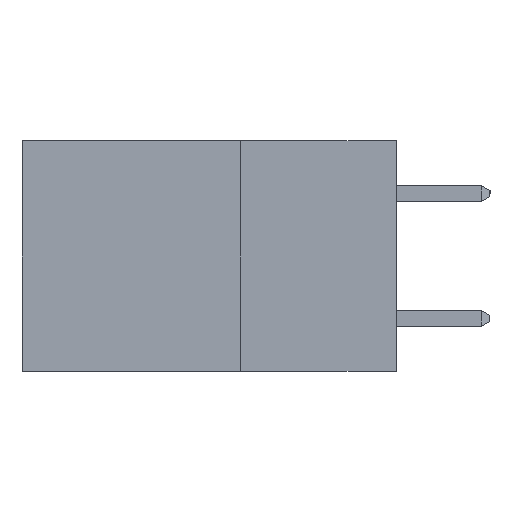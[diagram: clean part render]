
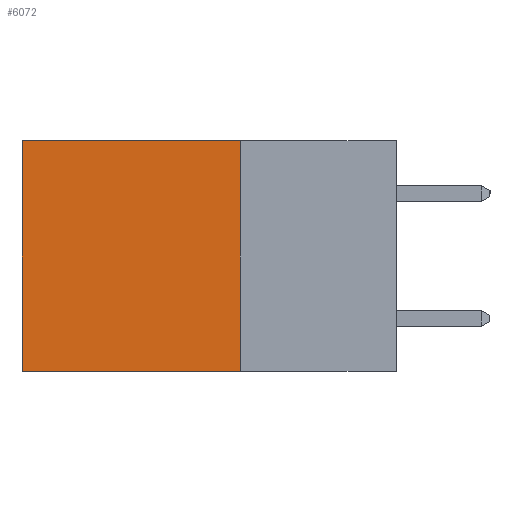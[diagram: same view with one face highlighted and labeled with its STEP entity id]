
A CAD part, left-side view. The second image highlights one B-rep face of the part: STEP entity #6072.
In plain terms, the highlighted planar face has unit normal (-1, 0, 0).
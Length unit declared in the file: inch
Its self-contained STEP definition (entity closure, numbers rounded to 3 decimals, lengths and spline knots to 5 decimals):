
#369 = DIRECTION ( 'NONE',  ( 1., 0., 0. ) ) ;
#497 = ORIENTED_EDGE ( 'NONE', *, *, #4588, .F. ) ;
#579 = LINE ( 'NONE', #3086, #5220 ) ;
#1056 = CARTESIAN_POINT ( 'NONE',  ( 0.2615, 0.25, 0. ) ) ;
#1070 = VERTEX_POINT ( 'NONE', #7358 ) ;
#2235 = PLANE ( 'NONE',  #9386 ) ;
#2494 = EDGE_CURVE ( 'NONE', #11170, #5965, #10393, .T. ) ;
#2817 = DIRECTION ( 'NONE',  ( 0., 1., 0. ) ) ;
#3086 = CARTESIAN_POINT ( 'NONE',  ( 0.2615, 0.6, -0.37 ) ) ;
#3148 = DIRECTION ( 'NONE',  ( 0., 0., -1. ) ) ;
#3241 = DIRECTION ( 'NONE',  ( 0., 0., -1. ) ) ;
#3710 = VECTOR ( 'NONE', #2817, 39.37008 ) ;
#4319 = CARTESIAN_POINT ( 'NONE',  ( 0.2615, 0.25, 0. ) ) ;
#4588 = EDGE_CURVE ( 'NONE', #5965, #1070, #8022, .T. ) ;
#4837 = EDGE_CURVE ( 'NONE', #11170, #6663, #10253, .T. ) ;
#4940 = DIRECTION ( 'NONE',  ( 0., 0., -1. ) ) ;
#5179 = DIRECTION ( 'NONE',  ( 0., 1., 0. ) ) ;
#5220 = VECTOR ( 'NONE', #3148, 39.37008 ) ;
#5713 = ORIENTED_EDGE ( 'NONE', *, *, #8676, .T. ) ;
#5965 = VERTEX_POINT ( 'NONE', #9864 ) ;
#6072 = ADVANCED_FACE ( 'NONE', ( #10201 ), #2235, .F. ) ;
#6257 = VECTOR ( 'NONE', #5179, 39.37008 ) ;
#6663 = VERTEX_POINT ( 'NONE', #9503 ) ;
#7358 = CARTESIAN_POINT ( 'NONE',  ( 0.2615, 0.6, -0.37 ) ) ;
#7450 = CARTESIAN_POINT ( 'NONE',  ( 0.2615, 0.25, -0.37 ) ) ;
#8022 = LINE ( 'NONE', #8079, #3710 ) ;
#8079 = CARTESIAN_POINT ( 'NONE',  ( 0.2615, 0.25, -0.37 ) ) ;
#8329 = EDGE_LOOP ( 'NONE', ( #5713, #497, #11009, #11025 ) ) ;
#8601 = VECTOR ( 'NONE', #3241, 39.37008 ) ;
#8676 = EDGE_CURVE ( 'NONE', #6663, #1070, #579, .T. ) ;
#9386 = AXIS2_PLACEMENT_3D ( 'NONE', #7450, #369, #4940 ) ;
#9503 = CARTESIAN_POINT ( 'NONE',  ( 0.2615, 0.6, 0. ) ) ;
#9864 = CARTESIAN_POINT ( 'NONE',  ( 0.2615, 0.25, -0.37 ) ) ;
#10201 = FACE_OUTER_BOUND ( 'NONE', #8329, .T. ) ;
#10223 = CARTESIAN_POINT ( 'NONE',  ( 0.2615, 0.25, -0.37 ) ) ;
#10253 = LINE ( 'NONE', #4319, #6257 ) ;
#10393 = LINE ( 'NONE', #10223, #8601 ) ;
#11009 = ORIENTED_EDGE ( 'NONE', *, *, #2494, .F. ) ;
#11025 = ORIENTED_EDGE ( 'NONE', *, *, #4837, .T. ) ;
#11170 = VERTEX_POINT ( 'NONE', #1056 ) ;
